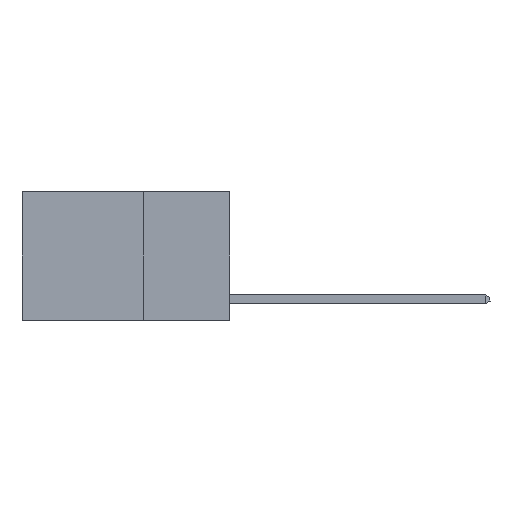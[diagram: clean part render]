
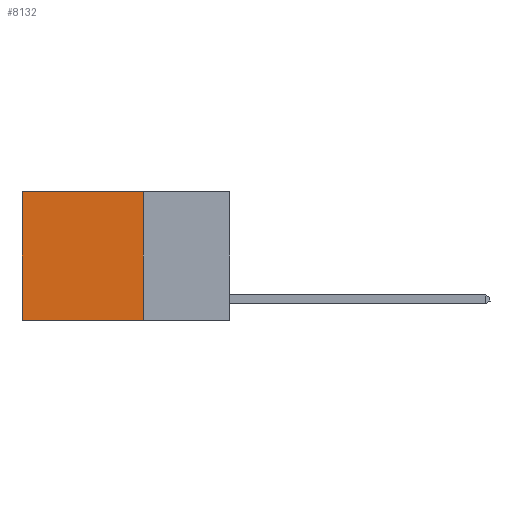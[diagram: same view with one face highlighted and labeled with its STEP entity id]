
A CAD part, left-side view. The second image highlights one B-rep face of the part: STEP entity #8132.
In plain terms, the highlighted planar face has unit normal (-1, 0, 0).
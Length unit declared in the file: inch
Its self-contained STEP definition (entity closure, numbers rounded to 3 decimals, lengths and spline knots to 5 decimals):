
#1078 = VECTOR ( 'NONE', #1246, 39.37008 ) ;
#1178 = CARTESIAN_POINT ( 'NONE',  ( 0.2625, 0.25, -0.37 ) ) ;
#1246 = DIRECTION ( 'NONE',  ( 0., 1., 0. ) ) ;
#1499 = EDGE_CURVE ( 'NONE', #2862, #5648, #2204, .T. ) ;
#1849 = VECTOR ( 'NONE', #6888, 39.37008 ) ;
#2204 = LINE ( 'NONE', #1178, #1849 ) ;
#2209 = CARTESIAN_POINT ( 'NONE',  ( 0.2625, 0.6, -0.37 ) ) ;
#2862 = VERTEX_POINT ( 'NONE', #11668 ) ;
#3031 = CARTESIAN_POINT ( 'NONE',  ( 0.2625, 0.6, 0. ) ) ;
#3167 = FACE_OUTER_BOUND ( 'NONE', #11156, .T. ) ;
#4192 = DIRECTION ( 'NONE',  ( 0., 0., -1. ) ) ;
#4556 = AXIS2_PLACEMENT_3D ( 'NONE', #12293, #5833, #13357 ) ;
#4568 = ORIENTED_EDGE ( 'NONE', *, *, #11354, .T. ) ;
#4712 = VERTEX_POINT ( 'NONE', #10510 ) ;
#5512 = CARTESIAN_POINT ( 'NONE',  ( 0.2625, 0.25, 0. ) ) ;
#5648 = VERTEX_POINT ( 'NONE', #2209 ) ;
#5833 = DIRECTION ( 'NONE',  ( 1., 0., 0. ) ) ;
#6486 = EDGE_CURVE ( 'NONE', #13741, #2862, #11613, .T. ) ;
#6888 = DIRECTION ( 'NONE',  ( 0., 1., 0. ) ) ;
#7185 = LINE ( 'NONE', #9128, #1078 ) ;
#7655 = CARTESIAN_POINT ( 'NONE',  ( 0.2625, 0.25, 0. ) ) ;
#8132 = ADVANCED_FACE ( 'NONE', ( #3167 ), #9048, .F. ) ;
#8332 = ORIENTED_EDGE ( 'NONE', *, *, #1499, .F. ) ;
#8746 = DIRECTION ( 'NONE',  ( 0., 0., -1. ) ) ;
#8982 = EDGE_CURVE ( 'NONE', #13741, #4712, #7185, .T. ) ;
#9048 = PLANE ( 'NONE',  #4556 ) ;
#9128 = CARTESIAN_POINT ( 'NONE',  ( 0.2625, 0.25, 0. ) ) ;
#9783 = ORIENTED_EDGE ( 'NONE', *, *, #6486, .F. ) ;
#9839 = VECTOR ( 'NONE', #4192, 39.37008 ) ;
#10431 = ORIENTED_EDGE ( 'NONE', *, *, #8982, .T. ) ;
#10510 = CARTESIAN_POINT ( 'NONE',  ( 0.2625, 0.6, 0. ) ) ;
#11156 = EDGE_LOOP ( 'NONE', ( #4568, #8332, #9783, #10431 ) ) ;
#11278 = VECTOR ( 'NONE', #8746, 39.37008 ) ;
#11354 = EDGE_CURVE ( 'NONE', #4712, #5648, #12985, .T. ) ;
#11613 = LINE ( 'NONE', #7655, #11278 ) ;
#11668 = CARTESIAN_POINT ( 'NONE',  ( 0.2625, 0.25, -0.37 ) ) ;
#12293 = CARTESIAN_POINT ( 'NONE',  ( 0.2625, 0.25, 0. ) ) ;
#12985 = LINE ( 'NONE', #3031, #9839 ) ;
#13357 = DIRECTION ( 'NONE',  ( 0., 0., -1. ) ) ;
#13741 = VERTEX_POINT ( 'NONE', #5512 ) ;
